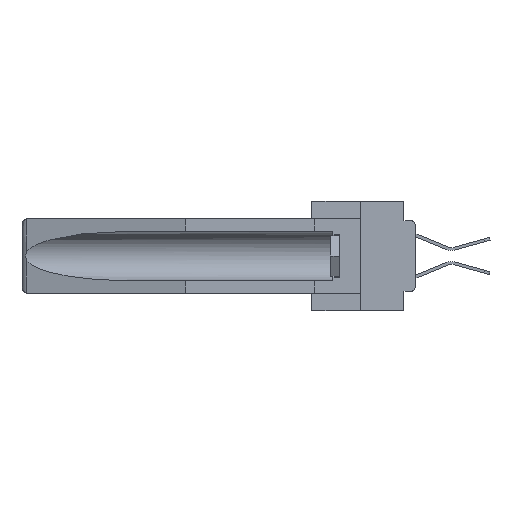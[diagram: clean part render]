
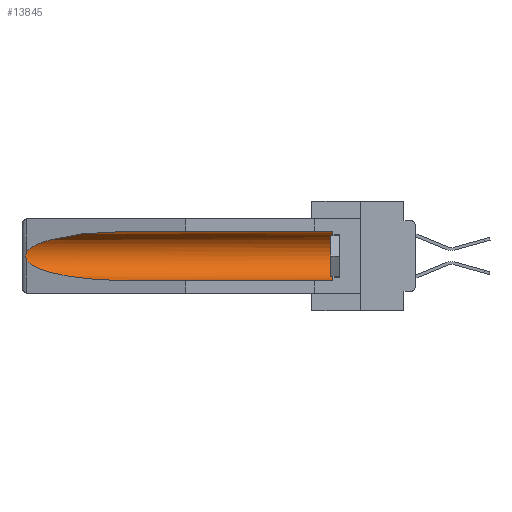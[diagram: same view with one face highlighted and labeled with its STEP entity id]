
A CAD part, left-side view. The second image highlights one B-rep face of the part: STEP entity #13845.
In plain terms, the highlighted cylindrical face has radius 2.857 mm (diameter 5.715 mm), a partial arc.
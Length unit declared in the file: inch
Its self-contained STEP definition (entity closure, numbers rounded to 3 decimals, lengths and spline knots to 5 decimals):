
#403 = CARTESIAN_POINT ( 'NONE',  ( 0.26537, 1.52718, -0.19328 ) ) ;
#587 = CARTESIAN_POINT ( 'NONE',  ( 0.26597, 1.5296, -0.19026 ) ) ;
#760 = LINE ( 'NONE', #14366, #27543 ) ;
#767 = CARTESIAN_POINT ( 'NONE',  ( 0.26654, 1.53092, -0.15636 ) ) ;
#938 = CARTESIAN_POINT ( 'NONE',  ( 0.21114, 1.30732, -0.284 ) ) ;
#1122 = CARTESIAN_POINT ( 'NONE',  ( 0.2675, 1.53308, -0.17534 ) ) ;
#1193 = ORIENTED_EDGE ( 'NONE', *, *, #6290, .T. ) ;
#1534 = CARTESIAN_POINT ( 'NONE',  ( 0.25451, 1.48313, -0.09465 ) ) ;
#1722 = CARTESIAN_POINT ( 'NONE',  ( 0.155, 1.07973, -0.059 ) ) ;
#1792 = ORIENTED_EDGE ( 'NONE', *, *, #17576, .T. ) ;
#2021 = VECTOR ( 'NONE', #13361, 39.37008 ) ;
#2328 = DIRECTION ( 'NONE',  ( 0., 1., 0. ) ) ;
#2458 = CARTESIAN_POINT ( 'NONE',  ( 0.155, -0.30754, -0.284 ) ) ;
#2867 = EDGE_CURVE ( 'NONE', #34275, #32925, #8526, .T. ) ;
#3608 = VERTEX_POINT ( 'NONE', #24132 ) ;
#3795 = CARTESIAN_POINT ( 'NONE',  ( 0.26597, 1.52961, -0.15275 ) ) ;
#3886 = AXIS2_PLACEMENT_3D ( 'NONE', #7861, #2328, #29505 ) ;
#6290 = EDGE_CURVE ( 'NONE', #3608, #8431, #15849, .T. ) ;
#6305 = CARTESIAN_POINT ( 'NONE',  ( 0.2673, 1.53269, -0.17917 ) ) ;
#7861 = CARTESIAN_POINT ( 'NONE',  ( 0.155, -0.30754, -0.1715 ) ) ;
#8047 = CYLINDRICAL_SURFACE ( 'NONE', #3886, 0.1125 ) ;
#8431 = VERTEX_POINT ( 'NONE', #29771 ) ;
#8526 =( BOUNDED_CURVE ( )  B_SPLINE_CURVE ( 3, ( #14377, #11675, #938, #9162 ),
 .UNSPECIFIED., .F., .F. ) 
 B_SPLINE_CURVE_WITH_KNOTS ( ( 4, 4 ),
 ( 0.1948, 1.5708 ),
 .UNSPECIFIED. ) 
 CURVE ( )  GEOMETRIC_REPRESENTATION_ITEM ( )  RATIONAL_B_SPLINE_CURVE ( ( 1., 0.848, 0.848, 1. ) ) 
 REPRESENTATION_ITEM ( '' )  );
#9162 = CARTESIAN_POINT ( 'NONE',  ( 0.155, 1.07973, -0.284 ) ) ;
#10469 = EDGE_CURVE ( 'NONE', #31711, #23288, #13240, .T. ) ;
#11675 = CARTESIAN_POINT ( 'NONE',  ( 0.25451, 1.48313, -0.24835 ) ) ;
#12077 = AXIS2_PLACEMENT_3D ( 'NONE', #15050, #25933, #14682 ) ;
#12549 = EDGE_LOOP ( 'NONE', ( #1193, #27802, #32755, #24797, #23062, #1792 ) ) ;
#13240 = CIRCLE ( 'NONE', #12077, 0.1125 ) ;
#13361 = DIRECTION ( 'NONE',  ( 0., 1., 0. ) ) ;
#13845 = ADVANCED_FACE ( 'NONE', ( #26835 ), #8047, .F. ) ;
#14007 = CARTESIAN_POINT ( 'NONE',  ( 0.2673, 1.5327, -0.16383 ) ) ;
#14174 = DIRECTION ( 'NONE',  ( 0., 1., 0. ) ) ;
#14366 = CARTESIAN_POINT ( 'NONE',  ( 0.155, -0.30754, -0.059 ) ) ;
#14377 = CARTESIAN_POINT ( 'NONE',  ( 0.26537, 1.52718, -0.19328 ) ) ;
#14682 = DIRECTION ( 'NONE',  ( 0., 0., 1. ) ) ;
#14713 = CARTESIAN_POINT ( 'NONE',  ( 0.26537, 1.52718, -0.14972 ) ) ;
#15050 = CARTESIAN_POINT ( 'NONE',  ( 0.155, 0.126, -0.1715 ) ) ;
#15849 =( BOUNDED_CURVE ( )  B_SPLINE_CURVE ( 3, ( #1722, #25863, #1534, #25501 ),
 .UNSPECIFIED., .F., .F. ) 
 B_SPLINE_CURVE_WITH_KNOTS ( ( 4, 4 ),
 ( 4.71239, 6.08839 ),
 .UNSPECIFIED. ) 
 CURVE ( )  GEOMETRIC_REPRESENTATION_ITEM ( )  RATIONAL_B_SPLINE_CURVE ( ( 1., 0.848, 0.848, 1. ) ) 
 REPRESENTATION_ITEM ( '' )  );
#16012 = CARTESIAN_POINT ( 'NONE',  ( 0.155, 0.126, -0.059 ) ) ;
#16099 = EDGE_CURVE ( 'NONE', #8431, #34275, #34684, .T. ) ;
#17228 = CARTESIAN_POINT ( 'NONE',  ( 0.26655, 1.53094, -0.18657 ) ) ;
#17576 = EDGE_CURVE ( 'NONE', #23288, #3608, #760, .T. ) ;
#21933 = CARTESIAN_POINT ( 'NONE',  ( 0.155, 0.126, -0.284 ) ) ;
#22577 = CARTESIAN_POINT ( 'NONE',  ( 0.2675, 1.53308, -0.16763 ) ) ;
#23062 = ORIENTED_EDGE ( 'NONE', *, *, #10469, .T. ) ;
#23288 = VERTEX_POINT ( 'NONE', #16012 ) ;
#23609 = CARTESIAN_POINT ( 'NONE',  ( 0.155, 1.07973, -0.284 ) ) ;
#24132 = CARTESIAN_POINT ( 'NONE',  ( 0.155, 1.07973, -0.059 ) ) ;
#24797 = ORIENTED_EDGE ( 'NONE', *, *, #30475, .F. ) ;
#25501 = CARTESIAN_POINT ( 'NONE',  ( 0.26537, 1.52718, -0.14972 ) ) ;
#25863 = CARTESIAN_POINT ( 'NONE',  ( 0.21114, 1.30732, -0.059 ) ) ;
#25933 = DIRECTION ( 'NONE',  ( 0., -1., 0. ) ) ;
#26835 = FACE_OUTER_BOUND ( 'NONE', #12549, .T. ) ;
#26972 = LINE ( 'NONE', #2458, #2021 ) ;
#27543 = VECTOR ( 'NONE', #14174, 39.37008 ) ;
#27802 = ORIENTED_EDGE ( 'NONE', *, *, #16099, .T. ) ;
#29505 = DIRECTION ( 'NONE',  ( 0., 0., 1. ) ) ;
#29771 = CARTESIAN_POINT ( 'NONE',  ( 0.26537, 1.52718, -0.14972 ) ) ;
#30475 = EDGE_CURVE ( 'NONE', #31711, #32925, #26972, .T. ) ;
#31711 = VERTEX_POINT ( 'NONE', #21933 ) ;
#32755 = ORIENTED_EDGE ( 'NONE', *, *, #2867, .T. ) ;
#32902 = CARTESIAN_POINT ( 'NONE',  ( 0.26537, 1.52718, -0.19328 ) ) ;
#32925 = VERTEX_POINT ( 'NONE', #23609 ) ;
#34275 = VERTEX_POINT ( 'NONE', #32902 ) ;
#34684 = B_SPLINE_CURVE_WITH_KNOTS ( 'NONE', 3,
 ( #14713, #3795, #767, #14007, #22577, #1122, #6305, #17228, #587, #403 ),
 .UNSPECIFIED., .F., .F.,
 ( 4, 2, 2, 2, 4 ),
 ( 0., 0.00029, 0.00058, 0.00087, 0.00117 ),
 .UNSPECIFIED. ) ;
